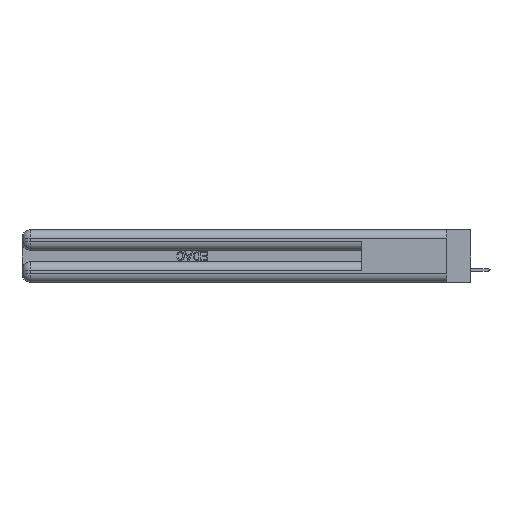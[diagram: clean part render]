
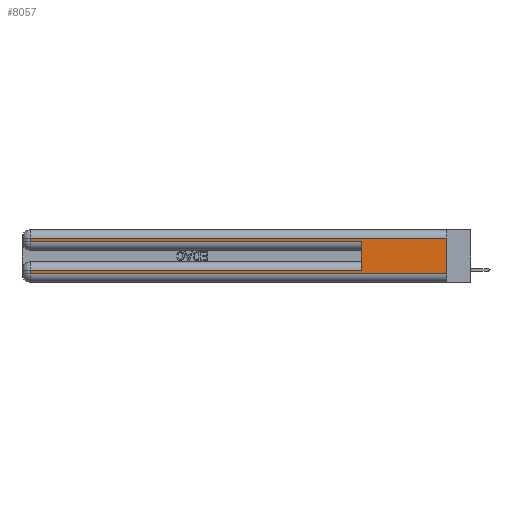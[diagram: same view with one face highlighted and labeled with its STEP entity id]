
A CAD part, left-side view. The second image highlights one B-rep face of the part: STEP entity #8057.
In plain terms, the highlighted planar face has unit normal (-1, 0, 0).
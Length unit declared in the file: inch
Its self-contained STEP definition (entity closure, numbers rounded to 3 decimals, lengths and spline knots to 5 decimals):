
#63 = EDGE_CURVE ( 'NONE', #27082, #39907, #22876, .T. ) ;
#338 = ORIENTED_EDGE ( 'NONE', *, *, #14727, .T. ) ;
#696 = CARTESIAN_POINT ( 'NONE',  ( 0., 0., 0.085 ) ) ;
#1395 = EDGE_LOOP ( 'NONE', ( #26299, #24947, #31017, #35135, #48908, #14109, #35629, #338 ) ) ;
#1660 = CARTESIAN_POINT ( 'NONE',  ( 0., 0.6, 0.145 ) ) ;
#1968 = LINE ( 'NONE', #39779, #8935 ) ;
#4312 = LINE ( 'NONE', #23702, #22676 ) ;
#5040 = VERTEX_POINT ( 'NONE', #32898 ) ;
#7163 = CARTESIAN_POINT ( 'NONE',  ( 0., 0.6, 0.085 ) ) ;
#7544 = CARTESIAN_POINT ( 'NONE',  ( 0., 2.94, 0.37 ) ) ;
#7599 = VERTEX_POINT ( 'NONE', #33810 ) ;
#8057 = ADVANCED_FACE ( 'NONE', ( #18812 ), #31530, .F. ) ;
#8542 = LINE ( 'NONE', #48101, #46615 ) ;
#8935 = VECTOR ( 'NONE', #22411, 39.37008 ) ;
#10679 = CARTESIAN_POINT ( 'NONE',  ( 0., 0., 0.06 ) ) ;
#12320 = VECTOR ( 'NONE', #22110, 39.37008 ) ;
#13416 = CARTESIAN_POINT ( 'NONE',  ( 0., 2.94, 0.31 ) ) ;
#14109 = ORIENTED_EDGE ( 'NONE', *, *, #24029, .T. ) ;
#14727 = EDGE_CURVE ( 'NONE', #7599, #43602, #1968, .T. ) ;
#15346 = CARTESIAN_POINT ( 'NONE',  ( 0., 0., 0.37 ) ) ;
#15565 = CARTESIAN_POINT ( 'NONE',  ( 0., 2.94, 0.085 ) ) ;
#16131 = EDGE_CURVE ( 'NONE', #32064, #43602, #4312, .T. ) ;
#16244 = EDGE_CURVE ( 'NONE', #5040, #39907, #40918, .T. ) ;
#17564 = CARTESIAN_POINT ( 'NONE',  ( 0., 0., 0.285 ) ) ;
#18812 = FACE_OUTER_BOUND ( 'NONE', #1395, .T. ) ;
#20751 = EDGE_CURVE ( 'NONE', #33879, #7599, #8542, .T. ) ;
#22110 = DIRECTION ( 'NONE',  ( 0., 0., 1. ) ) ;
#22411 = DIRECTION ( 'NONE',  ( 0., -1., 0. ) ) ;
#22676 = VECTOR ( 'NONE', #43860, 39.37008 ) ;
#22876 = LINE ( 'NONE', #1660, #12320 ) ;
#23271 = VECTOR ( 'NONE', #40835, 39.37008 ) ;
#23702 = CARTESIAN_POINT ( 'NONE',  ( 0., 0., 0.37 ) ) ;
#24029 = EDGE_CURVE ( 'NONE', #27082, #33879, #41016, .T. ) ;
#24483 = DIRECTION ( 'NONE',  ( 0., 0., -1. ) ) ;
#24947 = ORIENTED_EDGE ( 'NONE', *, *, #36544, .T. ) ;
#26299 = ORIENTED_EDGE ( 'NONE', *, *, #16131, .F. ) ;
#27082 = VERTEX_POINT ( 'NONE', #7163 ) ;
#29399 = VECTOR ( 'NONE', #41447, 39.37008 ) ;
#31017 = ORIENTED_EDGE ( 'NONE', *, *, #47650, .T. ) ;
#31530 = PLANE ( 'NONE',  #34951 ) ;
#31675 = LINE ( 'NONE', #7544, #50731 ) ;
#32064 = VERTEX_POINT ( 'NONE', #32791 ) ;
#32791 = CARTESIAN_POINT ( 'NONE',  ( 0., 0., 0.31 ) ) ;
#32898 = CARTESIAN_POINT ( 'NONE',  ( 0., 2.94, 0.285 ) ) ;
#32914 = DIRECTION ( 'NONE',  ( 0., 0., -1. ) ) ;
#33810 = CARTESIAN_POINT ( 'NONE',  ( 0., 2.94, 0.06 ) ) ;
#33879 = VERTEX_POINT ( 'NONE', #15565 ) ;
#34951 = AXIS2_PLACEMENT_3D ( 'NONE', #15346, #40000, #47725 ) ;
#35135 = ORIENTED_EDGE ( 'NONE', *, *, #16244, .T. ) ;
#35629 = ORIENTED_EDGE ( 'NONE', *, *, #20751, .T. ) ;
#36544 = EDGE_CURVE ( 'NONE', #32064, #48701, #45615, .T. ) ;
#36704 = VECTOR ( 'NONE', #37551, 39.37008 ) ;
#37551 = DIRECTION ( 'NONE',  ( 0., 1., 0. ) ) ;
#39779 = CARTESIAN_POINT ( 'NONE',  ( 0., 0., 0.06 ) ) ;
#39907 = VERTEX_POINT ( 'NONE', #44749 ) ;
#40000 = DIRECTION ( 'NONE',  ( 1., 0., 0. ) ) ;
#40835 = DIRECTION ( 'NONE',  ( 0., 1., 0. ) ) ;
#40918 = LINE ( 'NONE', #17564, #29399 ) ;
#41016 = LINE ( 'NONE', #696, #36704 ) ;
#41363 = CARTESIAN_POINT ( 'NONE',  ( 0., 0., 0.31 ) ) ;
#41447 = DIRECTION ( 'NONE',  ( 0., -1., 0. ) ) ;
#43602 = VERTEX_POINT ( 'NONE', #10679 ) ;
#43860 = DIRECTION ( 'NONE',  ( 0., 0., -1. ) ) ;
#44749 = CARTESIAN_POINT ( 'NONE',  ( 0., 0.6, 0.285 ) ) ;
#45615 = LINE ( 'NONE', #41363, #23271 ) ;
#46615 = VECTOR ( 'NONE', #24483, 39.37008 ) ;
#47650 = EDGE_CURVE ( 'NONE', #48701, #5040, #31675, .T. ) ;
#47725 = DIRECTION ( 'NONE',  ( 0., 0., -1. ) ) ;
#48101 = CARTESIAN_POINT ( 'NONE',  ( 0., 2.94, 0.37 ) ) ;
#48701 = VERTEX_POINT ( 'NONE', #13416 ) ;
#48908 = ORIENTED_EDGE ( 'NONE', *, *, #63, .F. ) ;
#50731 = VECTOR ( 'NONE', #32914, 39.37008 ) ;
